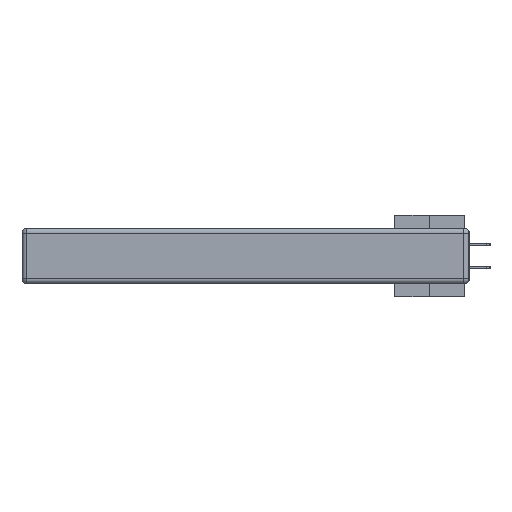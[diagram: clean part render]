
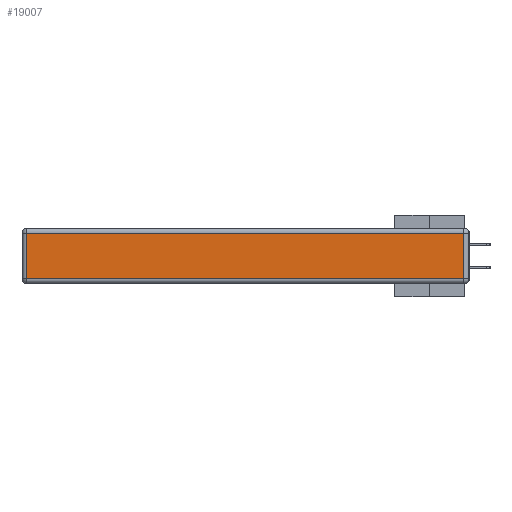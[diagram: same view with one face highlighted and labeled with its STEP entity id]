
A CAD part, left-side view. The second image highlights one B-rep face of the part: STEP entity #19007.
In plain terms, the highlighted planar face has unit normal (-1, 0, 0).
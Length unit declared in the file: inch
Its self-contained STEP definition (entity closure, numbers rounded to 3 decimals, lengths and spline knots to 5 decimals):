
#145 = CARTESIAN_POINT ( 'NONE',  ( 0., 0.03, -0.03 ) ) ;
#284 = AXIS2_PLACEMENT_3D ( 'NONE', #1811, #7584, #10753 ) ;
#733 = VERTEX_POINT ( 'NONE', #17065 ) ;
#1811 = CARTESIAN_POINT ( 'NONE',  ( 0., 0., -0.343 ) ) ;
#2541 = ORIENTED_EDGE ( 'NONE', *, *, #35032, .T. ) ;
#4885 = DIRECTION ( 'NONE',  ( 0., 1., 0. ) ) ;
#6780 = EDGE_CURVE ( 'NONE', #8269, #21434, #19359, .T. ) ;
#7008 = CARTESIAN_POINT ( 'NONE',  ( 0., 0., -0.313 ) ) ;
#7124 = DIRECTION ( 'NONE',  ( 0., -1., 0. ) ) ;
#7333 = LINE ( 'NONE', #18162, #8673 ) ;
#7584 = DIRECTION ( 'NONE',  ( -1., 0., 0. ) ) ;
#8269 = VERTEX_POINT ( 'NONE', #145 ) ;
#8673 = VECTOR ( 'NONE', #27778, 39.37008 ) ;
#9551 = VECTOR ( 'NONE', #28569, 39.37008 ) ;
#10048 = EDGE_LOOP ( 'NONE', ( #2541, #21043, #21022, #31019 ) ) ;
#10753 = DIRECTION ( 'NONE',  ( 0., 0., 1. ) ) ;
#11165 = CARTESIAN_POINT ( 'NONE',  ( 0., 2.72, -0.03 ) ) ;
#12762 = EDGE_CURVE ( 'NONE', #733, #8269, #19979, .T. ) ;
#13643 = PLANE ( 'NONE',  #284 ) ;
#16661 = CARTESIAN_POINT ( 'NONE',  ( 0., 2.75, -0.03 ) ) ;
#17065 = CARTESIAN_POINT ( 'NONE',  ( 0., 0.03, -0.313 ) ) ;
#18162 = CARTESIAN_POINT ( 'NONE',  ( 0., 2.72, -0.343 ) ) ;
#18831 = EDGE_CURVE ( 'NONE', #21434, #19479, #7333, .T. ) ;
#19007 = ADVANCED_FACE ( 'NONE', ( #22734 ), #13643, .T. ) ;
#19359 = LINE ( 'NONE', #16661, #20300 ) ;
#19479 = VERTEX_POINT ( 'NONE', #26815 ) ;
#19979 = LINE ( 'NONE', #25739, #9551 ) ;
#20300 = VECTOR ( 'NONE', #4885, 39.37008 ) ;
#21022 = ORIENTED_EDGE ( 'NONE', *, *, #6780, .T. ) ;
#21030 = LINE ( 'NONE', #7008, #28306 ) ;
#21043 = ORIENTED_EDGE ( 'NONE', *, *, #12762, .T. ) ;
#21434 = VERTEX_POINT ( 'NONE', #11165 ) ;
#22734 = FACE_OUTER_BOUND ( 'NONE', #10048, .T. ) ;
#25739 = CARTESIAN_POINT ( 'NONE',  ( 0., 0.03, -0.343 ) ) ;
#26815 = CARTESIAN_POINT ( 'NONE',  ( 0., 2.72, -0.313 ) ) ;
#27778 = DIRECTION ( 'NONE',  ( 0., 0., -1. ) ) ;
#28306 = VECTOR ( 'NONE', #7124, 39.37008 ) ;
#28569 = DIRECTION ( 'NONE',  ( 0., 0., 1. ) ) ;
#31019 = ORIENTED_EDGE ( 'NONE', *, *, #18831, .T. ) ;
#35032 = EDGE_CURVE ( 'NONE', #19479, #733, #21030, .T. ) ;
